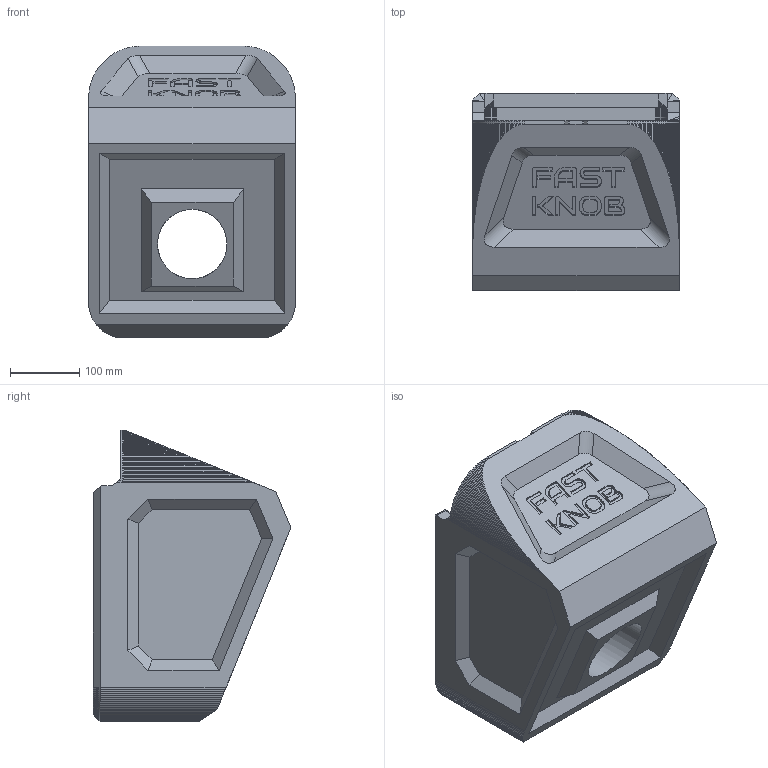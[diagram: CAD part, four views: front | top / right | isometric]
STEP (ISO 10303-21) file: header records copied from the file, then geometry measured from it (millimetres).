
FILE_DESCRIPTION(/* description */ (''),/* implementation_level */ '2;1');
FILE_NAME(/* name */ 'FAST KNOB.step',/* time_stamp */ '2021-06-01T09:45:06-06:00',/* author */ (''),/* organization */ (''),/* preprocessor_version */ 'ST-DEVELOPER v18.1',/* originating_system */ 'Autodesk Translation Framework v10.9.0.1377',/* authorisation */ '');
FILE_SCHEMA (('AUTOMOTIVE_DESIGN { 1 0 10303 214 3 1 1 }'));
Length unit declared in the file: millimetre
Products named in the file (1): FAST KNOB
Bounding box: 297.5 x 284.75 x 420 mm (x, y, z)
Volume: 18757768.8 mm3; surface area: 630126.7 mm2
Topology: 1 solids, 1 shells, 814 faces, 1956 edges, 1162 vertices
Faces by surface type: plane 684, bspline 125, cylinder 5
Full cylindrical faces by diameter (mm): 100 x1
Entity records: 22908 total; most frequent: CARTESIAN_POINT 5061, ORIENTED_EDGE 3912, DIRECTION 3133, EDGE_CURVE 1956, LINE 1657, VECTOR 1657, VERTEX_POINT 1162, EDGE_LOOP 834
